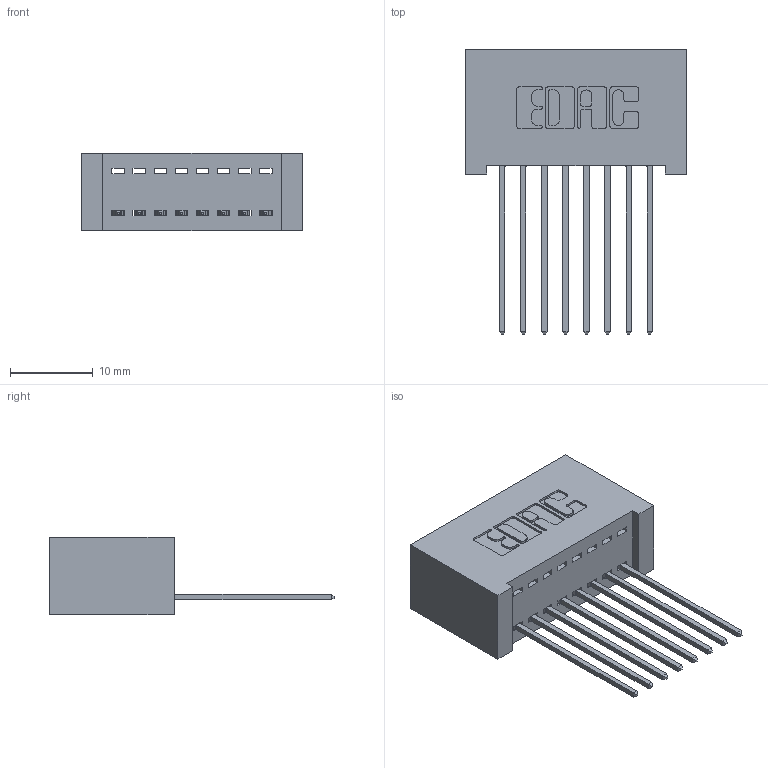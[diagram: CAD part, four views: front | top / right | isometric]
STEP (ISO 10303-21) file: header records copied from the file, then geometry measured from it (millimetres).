
FILE_DESCRIPTION (( 'STEP AP203' ), '1' );
FILE_NAME ('392-008-541-101.STEP', '2019-10-04T23:53:45', ( '' ), ( '' ), 'SwSTEP 2.0', 'SolidWorks 2016', '' );
FILE_SCHEMA (( 'CONFIG_CONTROL_DESIGN' ));
Length unit declared in the file: inch
Products named in the file (3): 342 Part_Lugless; 345-292-001_345-293-141; 392-008-541-101
Assembly tree (9 placements, depth 2):
  392-008-541-101
    342 Part_Lugless
    345-292-001_345-293-141  x8
Bounding box: 26.57 x 34.3 x 9.4 mm (x, y, z)
Volume: 2639.7 mm3; surface area: 3714.8 mm2
Topology: 9 solids, 9 shells, 566 faces, 1683 edges, 1110 vertices
Faces by surface type: plane 398, cylinder 168
Entity records: 8897 total; most frequent: CARTESIAN_POINT 1546, ORIENTED_EDGE 1490, DIRECTION 1365, EDGE_CURVE 745, LINE 625, VECTOR 625, VERTEX_POINT 494, AXIS2_PLACEMENT_3D 370
